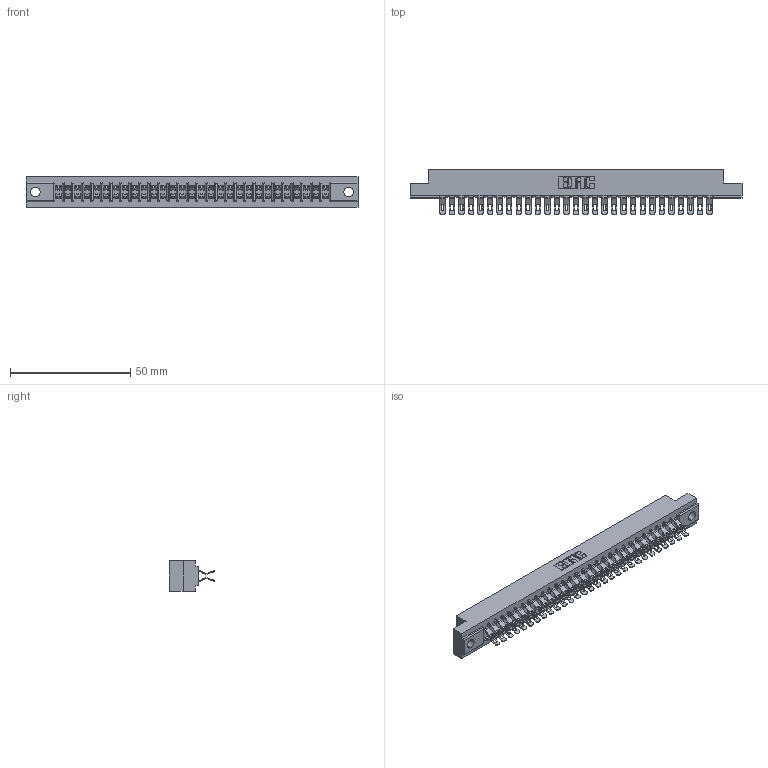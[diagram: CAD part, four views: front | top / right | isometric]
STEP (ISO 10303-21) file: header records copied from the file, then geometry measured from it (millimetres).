
FILE_DESCRIPTION (( 'STEP AP203' ), '1' );
FILE_NAME ('307-058-555-204.STEP', '2019-09-06T14:25:08', ( '' ), ( '' ), 'SwSTEP 2.0', 'SolidWorks 2016', '' );
FILE_SCHEMA (( 'CONFIG_CONTROL_DESIGN' ));
Length unit declared in the file: inch
Products named in the file (3): 307-058-555-204; 307 Part_.156 Dia Mounting Holes; 307-290-001_555
Assembly tree (59 placements, depth 2):
  307-058-555-204
    307 Part_.156 Dia Mounting Holes
    307-290-001_555  x58
Bounding box: 137.92 x 18.75 x 12.7 mm (x, y, z)
Volume: 14641.1 mm3; surface area: 18444.4 mm2
Topology: 59 solids, 59 shells, 3700 faces, 10857 edges, 7078 vertices
Faces by surface type: plane 2056, cylinder 1584, sphere 60
Entity records: 28347 total; most frequent: CARTESIAN_POINT 4651, ORIENTED_EDGE 4608, DIRECTION 4560, EDGE_CURVE 2304, VECTOR 1758, LINE 1758, VERTEX_POINT 1492, AXIS2_PLACEMENT_3D 1401
